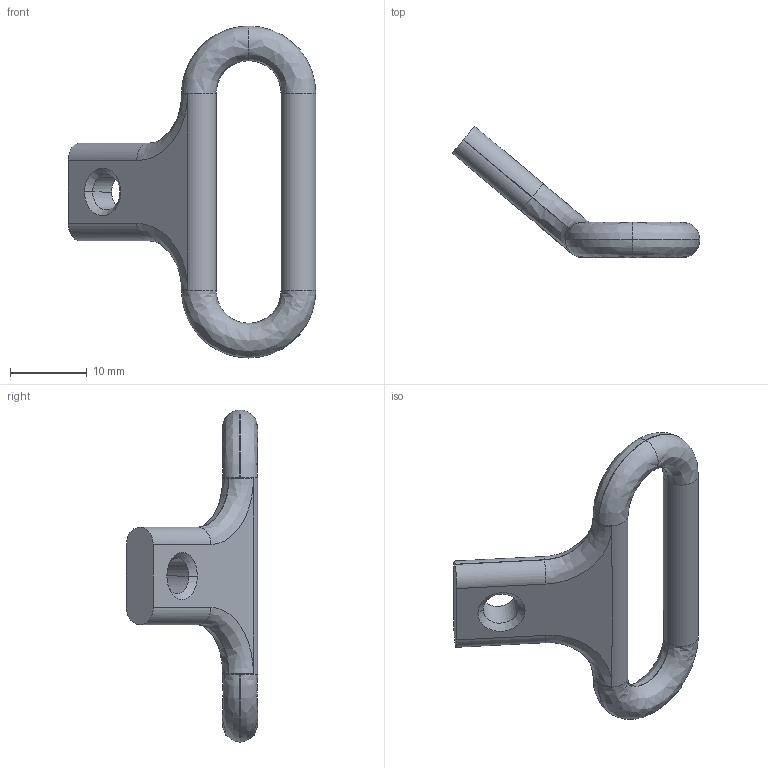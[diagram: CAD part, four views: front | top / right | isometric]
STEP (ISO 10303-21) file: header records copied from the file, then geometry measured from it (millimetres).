
FILE_DESCRIPTION (( 'STEP AP214' ), '1' );
FILE_NAME ('User Library-Telescopic Stock_Telescopic Stock Swivel1.STEP', '2013-05-23T12:55:55', ( 'Asher' ), ( '' ), 'SwSTEP 2.0', 'SolidWorks 2013', '' );
FILE_SCHEMA (( 'AUTOMOTIVE_DESIGN' ));
Length unit declared in the file: millimetre
Products named in the file (1): User Library-Telescopic Stock_Telescopic Stock Swivel1
Bounding box: 32.2 x 17.07 x 43.18 mm (x, y, z)
Volume: 2498.4 mm3; surface area: 1939.4 mm2
Topology: 1 solids, 1 shells, 42 faces, 102 edges, 60 vertices
Faces by surface type: cylinder 18, plane 12, bspline 10, cone 2
Entity records: 1490 total; most frequent: CARTESIAN_POINT 510, ORIENTED_EDGE 204, DIRECTION 182, EDGE_CURVE 102, AXIS2_PLACEMENT_3D 70, VERTEX_POINT 60, EDGE_LOOP 44, FACE_OUTER_BOUND 42
